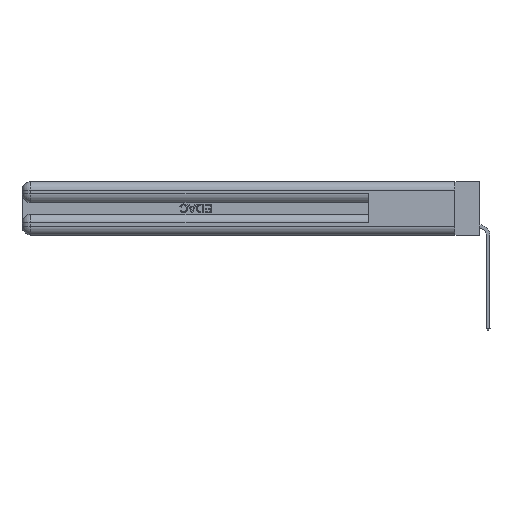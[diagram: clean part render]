
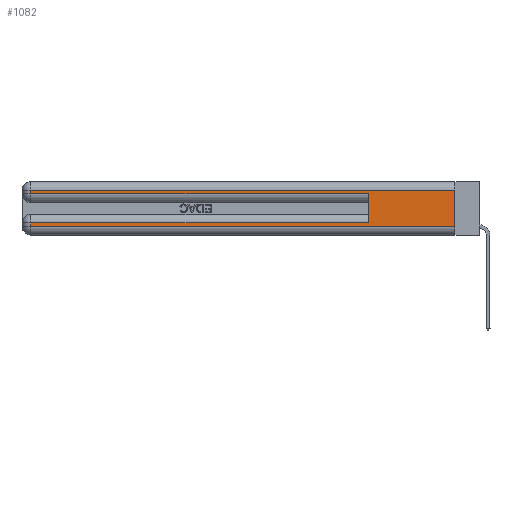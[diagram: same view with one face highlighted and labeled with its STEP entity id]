
A CAD part, left-side view. The second image highlights one B-rep face of the part: STEP entity #1082.
In plain terms, the highlighted planar face has unit normal (-1, 0, 0).
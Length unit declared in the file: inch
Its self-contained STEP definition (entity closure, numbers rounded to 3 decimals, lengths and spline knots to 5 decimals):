
#499 = VERTEX_POINT ( 'NONE', #1352 ) ;
#723 = ORIENTED_EDGE ( 'NONE', *, *, #21808, .F. ) ;
#1082 = ADVANCED_FACE ( 'NONE', ( #11983 ), #3545, .F. ) ;
#1093 = CARTESIAN_POINT ( 'NONE',  ( 0., 0., 0.06 ) ) ;
#1208 = VERTEX_POINT ( 'NONE', #1521 ) ;
#1273 = EDGE_CURVE ( 'NONE', #29526, #12247, #25608, .T. ) ;
#1352 = CARTESIAN_POINT ( 'NONE',  ( 0., 2.94, 0.285 ) ) ;
#1521 = CARTESIAN_POINT ( 'NONE',  ( 0., 2.94, 0.31 ) ) ;
#2533 = ORIENTED_EDGE ( 'NONE', *, *, #3962, .T. ) ;
#2592 = CARTESIAN_POINT ( 'NONE',  ( 0., 2.94, 0.085 ) ) ;
#3117 = VECTOR ( 'NONE', #21214, 39.37008 ) ;
#3545 = PLANE ( 'NONE',  #12738 ) ;
#3935 = VECTOR ( 'NONE', #5223, 39.37008 ) ;
#3962 = EDGE_CURVE ( 'NONE', #499, #5310, #10689, .T. ) ;
#4314 = CARTESIAN_POINT ( 'NONE',  ( 0., 2.94, 0.37 ) ) ;
#4789 = CARTESIAN_POINT ( 'NONE',  ( 0., 2.94, 0.06 ) ) ;
#4933 = CARTESIAN_POINT ( 'NONE',  ( 0., 0., 0.31 ) ) ;
#5223 = DIRECTION ( 'NONE',  ( 0., -1., 0. ) ) ;
#5310 = VERTEX_POINT ( 'NONE', #22303 ) ;
#5902 = ORIENTED_EDGE ( 'NONE', *, *, #26092, .T. ) ;
#6132 = CARTESIAN_POINT ( 'NONE',  ( 0., 0., 0.37 ) ) ;
#6428 = LINE ( 'NONE', #31401, #13114 ) ;
#6546 = CARTESIAN_POINT ( 'NONE',  ( 0., 2.94, 0.37 ) ) ;
#6808 = EDGE_CURVE ( 'NONE', #22333, #29526, #25713, .T. ) ;
#6894 = DIRECTION ( 'NONE',  ( 0., 0., -1. ) ) ;
#7700 = ORIENTED_EDGE ( 'NONE', *, *, #6808, .T. ) ;
#8636 = DIRECTION ( 'NONE',  ( 1., 0., 0. ) ) ;
#8693 = VECTOR ( 'NONE', #9896, 39.37008 ) ;
#9049 = EDGE_CURVE ( 'NONE', #20036, #1208, #6428, .T. ) ;
#9896 = DIRECTION ( 'NONE',  ( 0., 0., 1. ) ) ;
#10689 = LINE ( 'NONE', #17533, #3935 ) ;
#11579 = DIRECTION ( 'NONE',  ( 0., 0., -1. ) ) ;
#11983 = FACE_OUTER_BOUND ( 'NONE', #20542, .T. ) ;
#12247 = VERTEX_POINT ( 'NONE', #4789 ) ;
#12738 = AXIS2_PLACEMENT_3D ( 'NONE', #6132, #8636, #26081 ) ;
#13114 = VECTOR ( 'NONE', #16534, 39.37008 ) ;
#13262 = VECTOR ( 'NONE', #16222, 39.37008 ) ;
#15390 = LINE ( 'NONE', #29728, #8693 ) ;
#16222 = DIRECTION ( 'NONE',  ( 0., 1., 0. ) ) ;
#16534 = DIRECTION ( 'NONE',  ( 0., 1., 0. ) ) ;
#17533 = CARTESIAN_POINT ( 'NONE',  ( 0., 0., 0.285 ) ) ;
#17713 = EDGE_CURVE ( 'NONE', #1208, #499, #30644, .T. ) ;
#18953 = DIRECTION ( 'NONE',  ( 0., 0., -1. ) ) ;
#19802 = VECTOR ( 'NONE', #6894, 39.37008 ) ;
#20036 = VERTEX_POINT ( 'NONE', #4933 ) ;
#20542 = EDGE_LOOP ( 'NONE', ( #723, #26999, #25639, #2533, #21385, #7700, #28255, #5902 ) ) ;
#21214 = DIRECTION ( 'NONE',  ( 0., -1., 0. ) ) ;
#21385 = ORIENTED_EDGE ( 'NONE', *, *, #29978, .F. ) ;
#21459 = CARTESIAN_POINT ( 'NONE',  ( 0., 0., 0.37 ) ) ;
#21808 = EDGE_CURVE ( 'NONE', #20036, #23689, #30039, .T. ) ;
#22303 = CARTESIAN_POINT ( 'NONE',  ( 0., 0.6, 0.285 ) ) ;
#22333 = VERTEX_POINT ( 'NONE', #30953 ) ;
#23275 = VECTOR ( 'NONE', #11579, 39.37008 ) ;
#23441 = VECTOR ( 'NONE', #18953, 39.37008 ) ;
#23689 = VERTEX_POINT ( 'NONE', #26326 ) ;
#23918 = LINE ( 'NONE', #1093, #3117 ) ;
#25608 = LINE ( 'NONE', #4314, #19802 ) ;
#25639 = ORIENTED_EDGE ( 'NONE', *, *, #17713, .T. ) ;
#25713 = LINE ( 'NONE', #31088, #13262 ) ;
#26081 = DIRECTION ( 'NONE',  ( 0., 0., -1. ) ) ;
#26092 = EDGE_CURVE ( 'NONE', #12247, #23689, #23918, .T. ) ;
#26326 = CARTESIAN_POINT ( 'NONE',  ( 0., 0., 0.06 ) ) ;
#26999 = ORIENTED_EDGE ( 'NONE', *, *, #9049, .T. ) ;
#28255 = ORIENTED_EDGE ( 'NONE', *, *, #1273, .T. ) ;
#29526 = VERTEX_POINT ( 'NONE', #2592 ) ;
#29728 = CARTESIAN_POINT ( 'NONE',  ( 0., 0.6, 0.145 ) ) ;
#29978 = EDGE_CURVE ( 'NONE', #22333, #5310, #15390, .T. ) ;
#30039 = LINE ( 'NONE', #21459, #23441 ) ;
#30644 = LINE ( 'NONE', #6546, #23275 ) ;
#30953 = CARTESIAN_POINT ( 'NONE',  ( 0., 0.6, 0.085 ) ) ;
#31088 = CARTESIAN_POINT ( 'NONE',  ( 0., 0., 0.085 ) ) ;
#31401 = CARTESIAN_POINT ( 'NONE',  ( 0., 0., 0.31 ) ) ;
